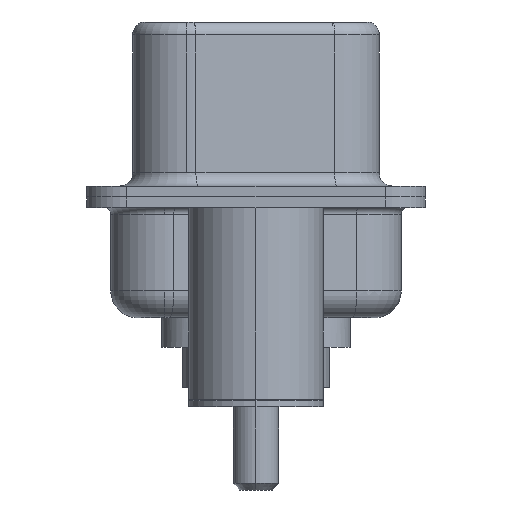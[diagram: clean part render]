
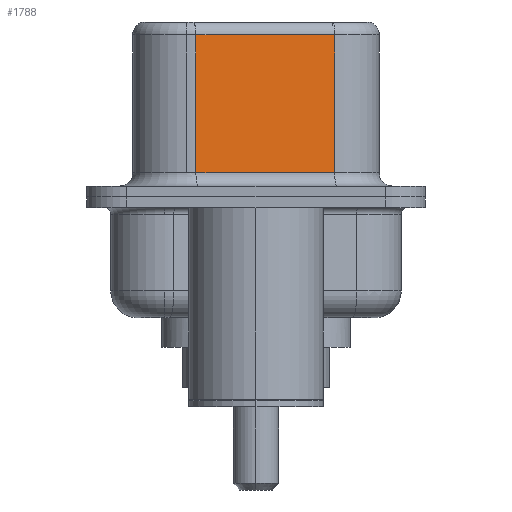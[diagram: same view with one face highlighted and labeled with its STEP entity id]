
A CAD part, left-side view. The second image highlights one B-rep face of the part: STEP entity #1788.
In plain terms, the highlighted planar face has unit normal (-0.985, -0.174, 0).
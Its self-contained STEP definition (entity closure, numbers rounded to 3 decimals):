
#211 = VERTEX_POINT ( 'NONE', #12852 ) ;
#402 = VECTOR ( 'NONE', #12418, 1000. ) ;
#453 = CARTESIAN_POINT ( 'NONE',  ( 4.58, -2.927, 6.02 ) ) ;
#622 = ORIENTED_EDGE ( 'NONE', *, *, #5015, .T. ) ;
#742 = DIRECTION ( 'NONE',  ( -0.174, 0.985, 0. ) ) ;
#1776 = VERTEX_POINT ( 'NONE', #16627 ) ;
#1788 = ADVANCED_FACE ( 'NONE', ( #16004 ), #3995, .F. ) ;
#2003 = LINE ( 'NONE', #453, #12091 ) ;
#2245 = CARTESIAN_POINT ( 'NONE',  ( 3.67, 2.233, 6.52 ) ) ;
#2546 = CARTESIAN_POINT ( 'NONE',  ( 4.58, -2.927, 6.02 ) ) ;
#2584 = CARTESIAN_POINT ( 'NONE',  ( 4.58, -2.927, 6.52 ) ) ;
#2814 = LINE ( 'NONE', #8553, #402 ) ;
#3995 = PLANE ( 'NONE',  #8439 ) ;
#4912 = ORIENTED_EDGE ( 'NONE', *, *, #5859, .T. ) ;
#5015 = EDGE_CURVE ( 'NONE', #211, #1776, #6840, .T. ) ;
#5304 = ORIENTED_EDGE ( 'NONE', *, *, #10116, .T. ) ;
#5724 = DIRECTION ( 'NONE',  ( 0., 0., -1. ) ) ;
#5859 = EDGE_CURVE ( 'NONE', #7525, #211, #2003, .T. ) ;
#6165 = EDGE_LOOP ( 'NONE', ( #14978, #4912, #622, #5304 ) ) ;
#6452 = VECTOR ( 'NONE', #8827, 1000. ) ;
#6840 = LINE ( 'NONE', #2245, #6452 ) ;
#7525 = VERTEX_POINT ( 'NONE', #2546 ) ;
#8439 = AXIS2_PLACEMENT_3D ( 'NONE', #2584, #9110, #15598 ) ;
#8553 = CARTESIAN_POINT ( 'NONE',  ( 4.58, -2.927, 0.9 ) ) ;
#8644 = VECTOR ( 'NONE', #5724, 1000. ) ;
#8827 = DIRECTION ( 'NONE',  ( 0., 0., -1. ) ) ;
#9110 = DIRECTION ( 'NONE',  ( 0.985, 0.174, 0. ) ) ;
#10116 = EDGE_CURVE ( 'NONE', #1776, #15330, #2814, .T. ) ;
#10892 = CARTESIAN_POINT ( 'NONE',  ( 4.58, -2.927, 6.52 ) ) ;
#12091 = VECTOR ( 'NONE', #742, 1000. ) ;
#12363 = CARTESIAN_POINT ( 'NONE',  ( 4.58, -2.927, 0.9 ) ) ;
#12418 = DIRECTION ( 'NONE',  ( 0.174, -0.985, 0. ) ) ;
#12588 = EDGE_CURVE ( 'NONE', #7525, #15330, #13474, .T. ) ;
#12852 = CARTESIAN_POINT ( 'NONE',  ( 3.67, 2.233, 6.02 ) ) ;
#13474 = LINE ( 'NONE', #10892, #8644 ) ;
#14978 = ORIENTED_EDGE ( 'NONE', *, *, #12588, .F. ) ;
#15330 = VERTEX_POINT ( 'NONE', #12363 ) ;
#15598 = DIRECTION ( 'NONE',  ( -0.174, 0.985, 0. ) ) ;
#16004 = FACE_OUTER_BOUND ( 'NONE', #6165, .T. ) ;
#16627 = CARTESIAN_POINT ( 'NONE',  ( 3.67, 2.233, 0.9 ) ) ;
